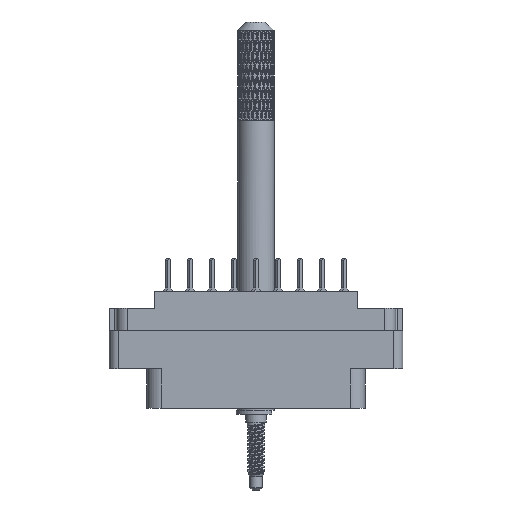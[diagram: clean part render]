
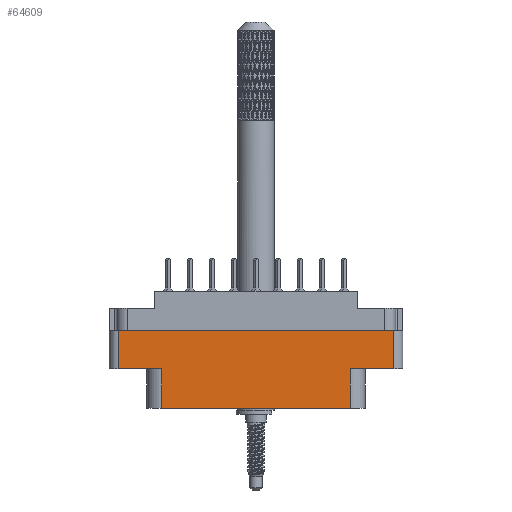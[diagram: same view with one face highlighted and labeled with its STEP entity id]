
A CAD part, front view. The second image highlights one B-rep face of the part: STEP entity #64609.
In plain terms, the highlighted planar face has unit normal (0, -1, 0).
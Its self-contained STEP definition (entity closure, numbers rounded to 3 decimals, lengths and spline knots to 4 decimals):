
#1531 = VERTEX_POINT ( 'NONE', #67377 ) ;
#3573 = ORIENTED_EDGE ( 'NONE', *, *, #36955, .F. ) ;
#4392 = EDGE_CURVE ( 'NONE', #52611, #1531, #67961, .T. ) ;
#4486 = CARTESIAN_POINT ( 'NONE',  ( -0.938, -0.438, -0.798 ) ) ;
#7579 = CARTESIAN_POINT ( 'NONE',  ( 0.644, -0.438, -0.529 ) ) ;
#8487 = LINE ( 'NONE', #4486, #90139 ) ;
#13407 = CARTESIAN_POINT ( 'NONE',  ( -0.644, -0.438, -0.798 ) ) ;
#14025 = CARTESIAN_POINT ( 'NONE',  ( 0.644, -0.438, -0.798 ) ) ;
#16560 = CARTESIAN_POINT ( 'NONE',  ( -0.938, -0.438, -0.268 ) ) ;
#19575 = EDGE_CURVE ( 'NONE', #76472, #97233, #8487, .T. ) ;
#21757 = CARTESIAN_POINT ( 'NONE',  ( 0., -0.438, -0.529 ) ) ;
#21761 = DIRECTION ( 'NONE',  ( 0., 0., 1. ) ) ;
#27740 = EDGE_CURVE ( 'NONE', #30451, #65508, #74785, .T. ) ;
#28205 = EDGE_CURVE ( 'NONE', #90619, #57627, #42642, .T. ) ;
#28815 = FACE_OUTER_BOUND ( 'NONE', #77689, .T. ) ;
#30246 = VECTOR ( 'NONE', #100786, 39.3701 ) ;
#30451 = VERTEX_POINT ( 'NONE', #16560 ) ;
#31056 = EDGE_CURVE ( 'NONE', #52611, #30451, #55954, .T. ) ;
#32765 = CARTESIAN_POINT ( 'NONE',  ( 0.938, -0.438, -0.268 ) ) ;
#36955 = EDGE_CURVE ( 'NONE', #57627, #97233, #63979, .T. ) ;
#42282 = CARTESIAN_POINT ( 'NONE',  ( -0.644, -0.438, -0.529 ) ) ;
#42415 = EDGE_CURVE ( 'NONE', #90619, #65508, #57092, .T. ) ;
#42642 = LINE ( 'NONE', #21757, #30246 ) ;
#42784 = ORIENTED_EDGE ( 'NONE', *, *, #4392, .T. ) ;
#44590 = DIRECTION ( 'NONE',  ( 1., 0., 0. ) ) ;
#46609 = VECTOR ( 'NONE', #92916, 39.3701 ) ;
#48830 = VECTOR ( 'NONE', #100245, 39.3701 ) ;
#51410 = PLANE ( 'NONE',  #60236 ) ;
#52320 = CARTESIAN_POINT ( 'NONE',  ( 0., -0.438, -0.529 ) ) ;
#52611 = VERTEX_POINT ( 'NONE', #83469 ) ;
#52735 = CARTESIAN_POINT ( 'NONE',  ( -1., -0.438, -0.268 ) ) ;
#53195 = ORIENTED_EDGE ( 'NONE', *, *, #27740, .F. ) ;
#53676 = DIRECTION ( 'NONE',  ( 1., 0., 0. ) ) ;
#54154 = DIRECTION ( 'NONE',  ( 0., 0., 1. ) ) ;
#55954 = LINE ( 'NONE', #100307, #69494 ) ;
#57092 = LINE ( 'NONE', #84649, #66970 ) ;
#57627 = VERTEX_POINT ( 'NONE', #7579 ) ;
#58192 = ORIENTED_EDGE ( 'NONE', *, *, #19575, .T. ) ;
#60236 = AXIS2_PLACEMENT_3D ( 'NONE', #75184, #83449, #66949 ) ;
#63979 = LINE ( 'NONE', #85304, #46609 ) ;
#64609 = ADVANCED_FACE ( 'NONE', ( #28815 ), #51410, .T. ) ;
#65508 = VERTEX_POINT ( 'NONE', #32765 ) ;
#66721 = ORIENTED_EDGE ( 'NONE', *, *, #74566, .T. ) ;
#66949 = DIRECTION ( 'NONE',  ( 0., 0., -1. ) ) ;
#66970 = VECTOR ( 'NONE', #21761, 39.3701 ) ;
#67121 = ORIENTED_EDGE ( 'NONE', *, *, #31056, .F. ) ;
#67377 = CARTESIAN_POINT ( 'NONE',  ( -0.644, -0.438, -0.529 ) ) ;
#67961 = LINE ( 'NONE', #52320, #80295 ) ;
#69494 = VECTOR ( 'NONE', #54154, 39.3701 ) ;
#71905 = ORIENTED_EDGE ( 'NONE', *, *, #42415, .T. ) ;
#73507 = CARTESIAN_POINT ( 'NONE',  ( 0.938, -0.438, -0.529 ) ) ;
#74566 = EDGE_CURVE ( 'NONE', #1531, #76472, #88224, .T. ) ;
#74785 = LINE ( 'NONE', #52735, #48830 ) ;
#75184 = CARTESIAN_POINT ( 'NONE',  ( -0.938, -0.438, -0.798 ) ) ;
#76472 = VERTEX_POINT ( 'NONE', #13407 ) ;
#77689 = EDGE_LOOP ( 'NONE', ( #66721, #58192, #3573, #98825, #71905, #53195, #67121, #42784 ) ) ;
#80295 = VECTOR ( 'NONE', #53676, 39.3701 ) ;
#83449 = DIRECTION ( 'NONE',  ( 0., -1., 0. ) ) ;
#83469 = CARTESIAN_POINT ( 'NONE',  ( -0.938, -0.438, -0.529 ) ) ;
#84649 = CARTESIAN_POINT ( 'NONE',  ( 0.938, -0.438, -0.798 ) ) ;
#85304 = CARTESIAN_POINT ( 'NONE',  ( 0.644, -0.438, -0.529 ) ) ;
#88224 = LINE ( 'NONE', #42282, #100509 ) ;
#89017 = DIRECTION ( 'NONE',  ( 0., 0., -1. ) ) ;
#90139 = VECTOR ( 'NONE', #44590, 39.3701 ) ;
#90619 = VERTEX_POINT ( 'NONE', #73507 ) ;
#92916 = DIRECTION ( 'NONE',  ( 0., 0., -1. ) ) ;
#97233 = VERTEX_POINT ( 'NONE', #14025 ) ;
#98825 = ORIENTED_EDGE ( 'NONE', *, *, #28205, .F. ) ;
#100245 = DIRECTION ( 'NONE',  ( 1., 0., 0. ) ) ;
#100307 = CARTESIAN_POINT ( 'NONE',  ( -0.938, -0.438, -0.798 ) ) ;
#100509 = VECTOR ( 'NONE', #89017, 39.3701 ) ;
#100786 = DIRECTION ( 'NONE',  ( -1., 0., 0. ) ) ;
